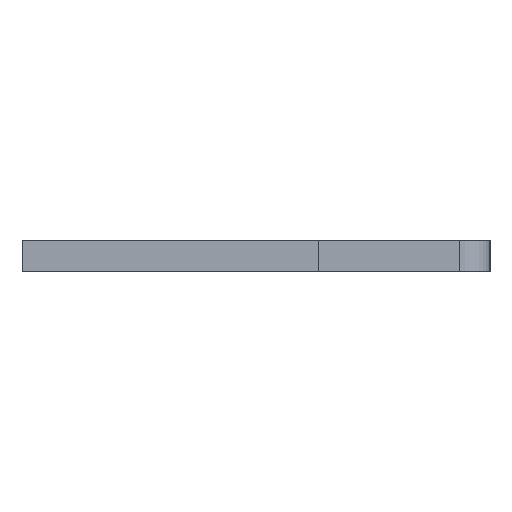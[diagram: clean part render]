
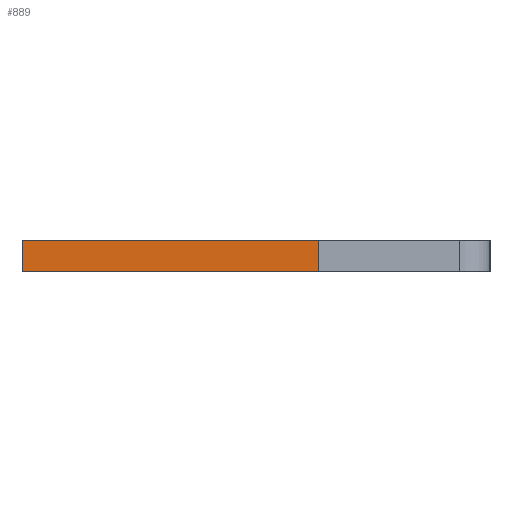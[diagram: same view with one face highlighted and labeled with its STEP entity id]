
A CAD part, left-side view. The second image highlights one B-rep face of the part: STEP entity #889.
In plain terms, the highlighted face is planar.
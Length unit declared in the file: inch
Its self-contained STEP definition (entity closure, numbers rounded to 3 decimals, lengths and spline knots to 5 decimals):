
#64 = PLANE ( 'NONE',  #1455 ) ;
#83 = VERTEX_POINT ( 'NONE', #1420 ) ;
#156 = ORIENTED_EDGE ( 'NONE', *, *, #1653, .F. ) ;
#205 = LINE ( 'NONE', #238, #673 ) ;
#206 = LINE ( 'NONE', #285, #329 ) ;
#238 = CARTESIAN_POINT ( 'NONE',  ( 0.01, -0.04, -0.04 ) ) ;
#244 = CARTESIAN_POINT ( 'NONE',  ( -0.01, 0.15, -0.04 ) ) ;
#285 = CARTESIAN_POINT ( 'NONE',  ( 0.01, 0.15, -0.04 ) ) ;
#329 = VECTOR ( 'NONE', #1237, 39.37008 ) ;
#375 = DIRECTION ( 'NONE',  ( 1., 0., 0. ) ) ;
#484 = EDGE_CURVE ( 'NONE', #2007, #83, #206, .T. ) ;
#552 = DIRECTION ( 'NONE',  ( -1., 0., 0. ) ) ;
#573 = LINE ( 'NONE', #1536, #907 ) ;
#574 = DIRECTION ( 'NONE',  ( -1., 0., 0. ) ) ;
#602 = FACE_OUTER_BOUND ( 'NONE', #967, .T. ) ;
#673 = VECTOR ( 'NONE', #552, 39.37008 ) ;
#773 = CARTESIAN_POINT ( 'NONE',  ( 0.01, -0.04, -0.04 ) ) ;
#862 = CARTESIAN_POINT ( 'NONE',  ( 0.01, 0.15, -0.04 ) ) ;
#889 = ADVANCED_FACE ( 'NONE', ( #602 ), #64, .F. ) ;
#903 = CARTESIAN_POINT ( 'NONE',  ( -0.01, -0.04, -0.04 ) ) ;
#907 = VECTOR ( 'NONE', #574, 39.37008 ) ;
#915 = CARTESIAN_POINT ( 'NONE',  ( -0.01, 0.15, -0.04 ) ) ;
#967 = EDGE_LOOP ( 'NONE', ( #1805, #156, #1259, #1421 ) ) ;
#1208 = EDGE_CURVE ( 'NONE', #2007, #1777, #205, .T. ) ;
#1232 = DIRECTION ( 'NONE',  ( 0., 1., 0. ) ) ;
#1237 = DIRECTION ( 'NONE',  ( 0., 1., 0. ) ) ;
#1259 = ORIENTED_EDGE ( 'NONE', *, *, #484, .F. ) ;
#1305 = EDGE_CURVE ( 'NONE', #1777, #1650, #1648, .T. ) ;
#1420 = CARTESIAN_POINT ( 'NONE',  ( 0.01, 0.15, -0.04 ) ) ;
#1421 = ORIENTED_EDGE ( 'NONE', *, *, #1208, .T. ) ;
#1455 = AXIS2_PLACEMENT_3D ( 'NONE', #862, #1508, #375 ) ;
#1508 = DIRECTION ( 'NONE',  ( 0., 0., 1. ) ) ;
#1536 = CARTESIAN_POINT ( 'NONE',  ( 0.01, 0.15, -0.04 ) ) ;
#1648 = LINE ( 'NONE', #244, #1880 ) ;
#1650 = VERTEX_POINT ( 'NONE', #915 ) ;
#1653 = EDGE_CURVE ( 'NONE', #83, #1650, #573, .T. ) ;
#1777 = VERTEX_POINT ( 'NONE', #903 ) ;
#1805 = ORIENTED_EDGE ( 'NONE', *, *, #1305, .T. ) ;
#1880 = VECTOR ( 'NONE', #1232, 39.37008 ) ;
#2007 = VERTEX_POINT ( 'NONE', #773 ) ;
